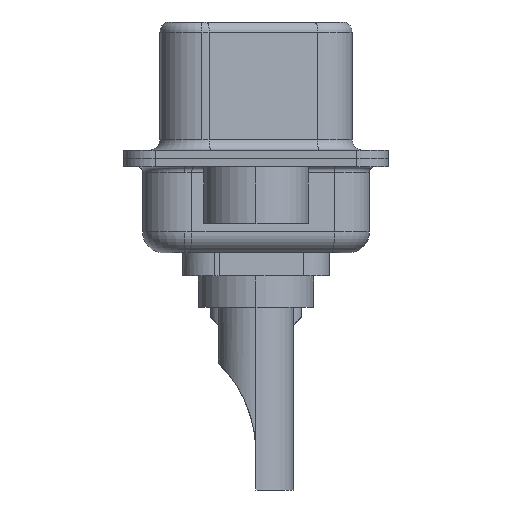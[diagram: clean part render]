
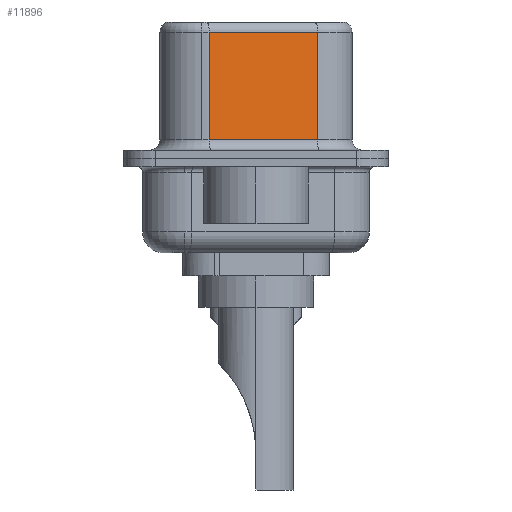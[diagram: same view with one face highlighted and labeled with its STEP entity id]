
A CAD part, left-side view. The second image highlights one B-rep face of the part: STEP entity #11896.
In plain terms, the highlighted planar face has unit normal (-0.985, -0.174, 0).
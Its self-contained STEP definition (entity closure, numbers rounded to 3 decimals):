
#182 = VECTOR ( 'NONE', #12314, 1000. ) ;
#293 = VECTOR ( 'NONE', #3204, 1000. ) ;
#1238 = CARTESIAN_POINT ( 'NONE',  ( 4.585, -2.927, 6.02 ) ) ;
#1701 = CARTESIAN_POINT ( 'NONE',  ( 4.585, -2.927, 0.9 ) ) ;
#1816 = VERTEX_POINT ( 'NONE', #1910 ) ;
#1910 = CARTESIAN_POINT ( 'NONE',  ( 3.675, 2.233, 0.9 ) ) ;
#2363 = ORIENTED_EDGE ( 'NONE', *, *, #2916, .T. ) ;
#2916 = EDGE_CURVE ( 'NONE', #7243, #1816, #4348, .T. ) ;
#3192 = EDGE_CURVE ( 'NONE', #10907, #7243, #18899, .T. ) ;
#3204 = DIRECTION ( 'NONE',  ( 0., 0., -1. ) ) ;
#4348 = LINE ( 'NONE', #5367, #293 ) ;
#5074 = EDGE_CURVE ( 'NONE', #10907, #18766, #11929, .T. ) ;
#5367 = CARTESIAN_POINT ( 'NONE',  ( 3.675, 2.233, 6.52 ) ) ;
#5586 = ORIENTED_EDGE ( 'NONE', *, *, #11706, .T. ) ;
#6707 = CARTESIAN_POINT ( 'NONE',  ( 4.585, -2.927, 6.52 ) ) ;
#7243 = VERTEX_POINT ( 'NONE', #9069 ) ;
#7778 = CARTESIAN_POINT ( 'NONE',  ( 4.585, -2.927, 0.9 ) ) ;
#7872 = VECTOR ( 'NONE', #8582, 1000. ) ;
#8309 = CARTESIAN_POINT ( 'NONE',  ( 4.585, -2.927, 6.52 ) ) ;
#8582 = DIRECTION ( 'NONE',  ( 0., 0., -1. ) ) ;
#9069 = CARTESIAN_POINT ( 'NONE',  ( 3.675, 2.233, 6.02 ) ) ;
#9848 = DIRECTION ( 'NONE',  ( -0.174, 0.985, 0. ) ) ;
#10090 = CARTESIAN_POINT ( 'NONE',  ( 4.585, -2.927, 6.02 ) ) ;
#10282 = AXIS2_PLACEMENT_3D ( 'NONE', #8309, #18961, #9848 ) ;
#10816 = VECTOR ( 'NONE', #18236, 1000. ) ;
#10907 = VERTEX_POINT ( 'NONE', #1238 ) ;
#11430 = LINE ( 'NONE', #7778, #182 ) ;
#11706 = EDGE_CURVE ( 'NONE', #1816, #18766, #11430, .T. ) ;
#11896 = ADVANCED_FACE ( 'NONE', ( #12601 ), #17432, .F. ) ;
#11929 = LINE ( 'NONE', #6707, #7872 ) ;
#12314 = DIRECTION ( 'NONE',  ( 0.174, -0.985, 0. ) ) ;
#12601 = FACE_OUTER_BOUND ( 'NONE', #16879, .T. ) ;
#16879 = EDGE_LOOP ( 'NONE', ( #17949, #17911, #2363, #5586 ) ) ;
#17432 = PLANE ( 'NONE',  #10282 ) ;
#17911 = ORIENTED_EDGE ( 'NONE', *, *, #3192, .T. ) ;
#17949 = ORIENTED_EDGE ( 'NONE', *, *, #5074, .F. ) ;
#18236 = DIRECTION ( 'NONE',  ( -0.174, 0.985, 0. ) ) ;
#18766 = VERTEX_POINT ( 'NONE', #1701 ) ;
#18899 = LINE ( 'NONE', #10090, #10816 ) ;
#18961 = DIRECTION ( 'NONE',  ( 0.985, 0.174, 0. ) ) ;
